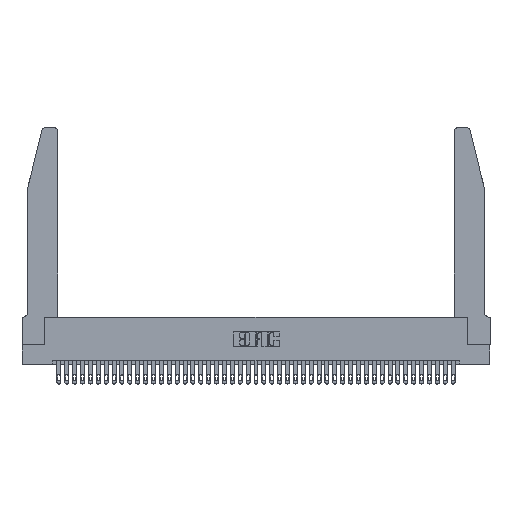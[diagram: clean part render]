
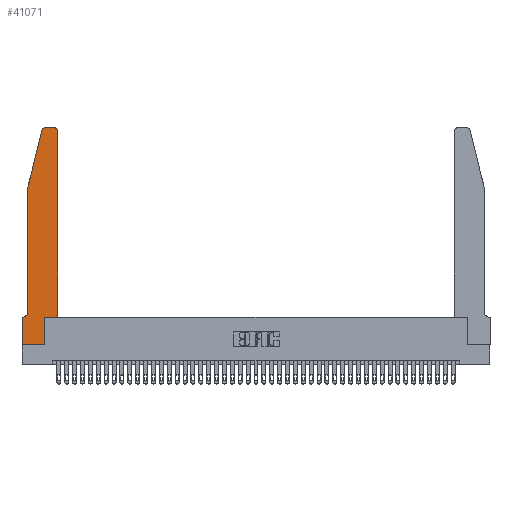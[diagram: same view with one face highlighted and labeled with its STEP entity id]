
A CAD part, top view. The second image highlights one B-rep face of the part: STEP entity #41071.
In plain terms, the highlighted planar face has unit normal (0, 0, 1).
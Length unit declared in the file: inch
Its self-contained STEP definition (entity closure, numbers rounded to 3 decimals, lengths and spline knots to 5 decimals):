
#484 = VERTEX_POINT ( 'NONE', #26643 ) ;
#717 = CARTESIAN_POINT ( 'NONE',  ( 0.4205, 2.75, 0.37 ) ) ;
#905 = VERTEX_POINT ( 'NONE', #717 ) ;
#1379 = ORIENTED_EDGE ( 'NONE', *, *, #9922, .T. ) ;
#1496 = VERTEX_POINT ( 'NONE', #21116 ) ;
#1949 = EDGE_CURVE ( 'NONE', #31339, #36221, #4055, .T. ) ;
#2039 = VERTEX_POINT ( 'NONE', #7175 ) ;
#2255 = DIRECTION ( 'NONE',  ( -1., 0., 0. ) ) ;
#2691 = VECTOR ( 'NONE', #29143, 39.37008 ) ;
#3434 = EDGE_CURVE ( 'NONE', #1496, #10016, #9019, .T. ) ;
#3852 = CARTESIAN_POINT ( 'NONE',  ( 0.4205, 2.72, 0.37 ) ) ;
#4055 = LINE ( 'NONE', #26378, #25568 ) ;
#4882 = ORIENTED_EDGE ( 'NONE', *, *, #3434, .T. ) ;
#5181 = DIRECTION ( 'NONE',  ( 0., 1., 0. ) ) ;
#5327 = CARTESIAN_POINT ( 'NONE',  ( 0.2605, 2.75, 0.37 ) ) ;
#5723 = DIRECTION ( 'NONE',  ( 0., 0., 1. ) ) ;
#6067 = ORIENTED_EDGE ( 'NONE', *, *, #11130, .T. ) ;
#6348 = DIRECTION ( 'NONE',  ( -1., 0., 0. ) ) ;
#6648 = CARTESIAN_POINT ( 'NONE',  ( 0.0755, 2., 0.37 ) ) ;
#6982 = EDGE_CURVE ( 'NONE', #36221, #2039, #8767, .T. ) ;
#7175 = CARTESIAN_POINT ( 'NONE',  ( 0., 0., 0.37 ) ) ;
#7281 = ORIENTED_EDGE ( 'NONE', *, *, #27553, .T. ) ;
#8188 = ORIENTED_EDGE ( 'NONE', *, *, #40247, .T. ) ;
#8767 = LINE ( 'NONE', #36379, #34477 ) ;
#9019 = LINE ( 'NONE', #13592, #17405 ) ;
#9922 = EDGE_CURVE ( 'NONE', #17759, #40126, #40561, .T. ) ;
#10016 = VERTEX_POINT ( 'NONE', #13147 ) ;
#10155 = EDGE_LOOP ( 'NONE', ( #14805, #6067, #34357, #1379, #36554, #12082, #42705, #31238, #13639, #8188, #4882, #7281 ) ) ;
#11130 = EDGE_CURVE ( 'NONE', #484, #39141, #29156, .T. ) ;
#11888 = CARTESIAN_POINT ( 'NONE',  ( 0.4505, 0.35, 0.37 ) ) ;
#11921 = CARTESIAN_POINT ( 'NONE',  ( 0.284, 2.72, 0.37 ) ) ;
#12082 = ORIENTED_EDGE ( 'NONE', *, *, #1949, .T. ) ;
#12942 = DIRECTION ( 'NONE',  ( 0., 0., -1. ) ) ;
#13147 = CARTESIAN_POINT ( 'NONE',  ( 0.4505, 2.72, 0.37 ) ) ;
#13240 = DIRECTION ( 'NONE',  ( 0., 0., 1. ) ) ;
#13265 = LINE ( 'NONE', #38391, #28502 ) ;
#13366 = CARTESIAN_POINT ( 'NONE',  ( 0.0755, 2., 0.37 ) ) ;
#13396 = DIRECTION ( 'NONE',  ( -0.239, -0.971, 0. ) ) ;
#13481 = EDGE_CURVE ( 'NONE', #39141, #17759, #31474, .T. ) ;
#13592 = CARTESIAN_POINT ( 'NONE',  ( 0.4505, 0.35, 0.37 ) ) ;
#13639 = ORIENTED_EDGE ( 'NONE', *, *, #17603, .T. ) ;
#13683 = DIRECTION ( 'NONE',  ( 1., 0., 0. ) ) ;
#14805 = ORIENTED_EDGE ( 'NONE', *, *, #32556, .T. ) ;
#14888 = VECTOR ( 'NONE', #19567, 39.37008 ) ;
#15300 = AXIS2_PLACEMENT_3D ( 'NONE', #11921, #22026, #42054 ) ;
#16085 = CARTESIAN_POINT ( 'NONE',  ( 0.0755, 2., 0.37 ) ) ;
#17405 = VECTOR ( 'NONE', #23979, 39.37008 ) ;
#17603 = EDGE_CURVE ( 'NONE', #35382, #36583, #13265, .T. ) ;
#17759 = VERTEX_POINT ( 'NONE', #13366 ) ;
#19110 = CIRCLE ( 'NONE', #40493, 0.07 ) ;
#19567 = DIRECTION ( 'NONE',  ( 1., 0., 0. ) ) ;
#19771 = DIRECTION ( 'NONE',  ( -1., 0., 0. ) ) ;
#20190 = CARTESIAN_POINT ( 'NONE',  ( 0.2865, 0.35, 0.37 ) ) ;
#20247 = VECTOR ( 'NONE', #35393, 39.37008 ) ;
#20438 = AXIS2_PLACEMENT_3D ( 'NONE', #3852, #13240, #13683 ) ;
#20755 = AXIS2_PLACEMENT_3D ( 'NONE', #36133, #5723, #25690 ) ;
#21116 = CARTESIAN_POINT ( 'NONE',  ( 0.4505, 0.35, 0.37 ) ) ;
#21182 = LINE ( 'NONE', #29834, #14888 ) ;
#22026 = DIRECTION ( 'NONE',  ( 0., 0., 1. ) ) ;
#23979 = DIRECTION ( 'NONE',  ( 0., 1., 0. ) ) ;
#25209 = VECTOR ( 'NONE', #13396, 39.37008 ) ;
#25568 = VECTOR ( 'NONE', #19771, 39.37008 ) ;
#25690 = DIRECTION ( 'NONE',  ( 1., 0., 0. ) ) ;
#26193 = CARTESIAN_POINT ( 'NONE',  ( 0.25487, 2.72718, 0.37 ) ) ;
#26378 = CARTESIAN_POINT ( 'NONE',  ( 0.0755, 0.35, 0.37 ) ) ;
#26643 = CARTESIAN_POINT ( 'NONE',  ( 0.284, 2.75, 0.37 ) ) ;
#27553 = EDGE_CURVE ( 'NONE', #10016, #905, #35145, .T. ) ;
#27730 = CARTESIAN_POINT ( 'NONE',  ( 0.0755, 0.42, 0.37 ) ) ;
#28502 = VECTOR ( 'NONE', #5181, 39.37008 ) ;
#28542 = FACE_OUTER_BOUND ( 'NONE', #10155, .T. ) ;
#29143 = DIRECTION ( 'NONE',  ( 0., -1., 0. ) ) ;
#29156 = CIRCLE ( 'NONE', #15300, 0.03 ) ;
#29834 = CARTESIAN_POINT ( 'NONE',  ( 0., 0., 0.37 ) ) ;
#29875 = VECTOR ( 'NONE', #2255, 39.37008 ) ;
#31238 = ORIENTED_EDGE ( 'NONE', *, *, #34000, .T. ) ;
#31339 = VERTEX_POINT ( 'NONE', #31994 ) ;
#31474 = LINE ( 'NONE', #6648, #25209 ) ;
#31994 = CARTESIAN_POINT ( 'NONE',  ( 0.0055, 0.35, 0.37 ) ) ;
#32556 = EDGE_CURVE ( 'NONE', #905, #484, #40431, .T. ) ;
#32724 = PLANE ( 'NONE',  #20755 ) ;
#34000 = EDGE_CURVE ( 'NONE', #2039, #35382, #21182, .T. ) ;
#34357 = ORIENTED_EDGE ( 'NONE', *, *, #13481, .T. ) ;
#34477 = VECTOR ( 'NONE', #39742, 39.37008 ) ;
#35145 = CIRCLE ( 'NONE', #20438, 0.03 ) ;
#35382 = VERTEX_POINT ( 'NONE', #43385 ) ;
#35393 = DIRECTION ( 'NONE',  ( 1., 0., 0. ) ) ;
#35496 = LINE ( 'NONE', #11888, #20247 ) ;
#36133 = CARTESIAN_POINT ( 'NONE',  ( 0., 0.35, 0.37 ) ) ;
#36221 = VERTEX_POINT ( 'NONE', #38633 ) ;
#36379 = CARTESIAN_POINT ( 'NONE',  ( 0., 0., 0.37 ) ) ;
#36554 = ORIENTED_EDGE ( 'NONE', *, *, #40848, .T. ) ;
#36583 = VERTEX_POINT ( 'NONE', #20190 ) ;
#38391 = CARTESIAN_POINT ( 'NONE',  ( 0.2865, 0.35, 0.37 ) ) ;
#38633 = CARTESIAN_POINT ( 'NONE',  ( 0., 0.35, 0.37 ) ) ;
#39141 = VERTEX_POINT ( 'NONE', #26193 ) ;
#39327 = CARTESIAN_POINT ( 'NONE',  ( 0.0055, 0.42, 0.37 ) ) ;
#39742 = DIRECTION ( 'NONE',  ( 0., -1., 0. ) ) ;
#40126 = VERTEX_POINT ( 'NONE', #27730 ) ;
#40247 = EDGE_CURVE ( 'NONE', #36583, #1496, #35496, .T. ) ;
#40431 = LINE ( 'NONE', #5327, #29875 ) ;
#40493 = AXIS2_PLACEMENT_3D ( 'NONE', #39327, #12942, #6348 ) ;
#40561 = LINE ( 'NONE', #16085, #2691 ) ;
#40848 = EDGE_CURVE ( 'NONE', #40126, #31339, #19110, .T. ) ;
#41071 = ADVANCED_FACE ( 'NONE', ( #28542 ), #32724, .T. ) ;
#42054 = DIRECTION ( 'NONE',  ( 1., 0., 0. ) ) ;
#42705 = ORIENTED_EDGE ( 'NONE', *, *, #6982, .T. ) ;
#43385 = CARTESIAN_POINT ( 'NONE',  ( 0.2865, 0., 0.37 ) ) ;
